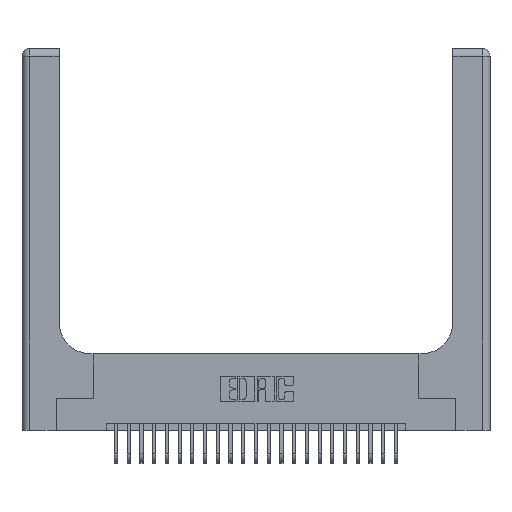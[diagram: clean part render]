
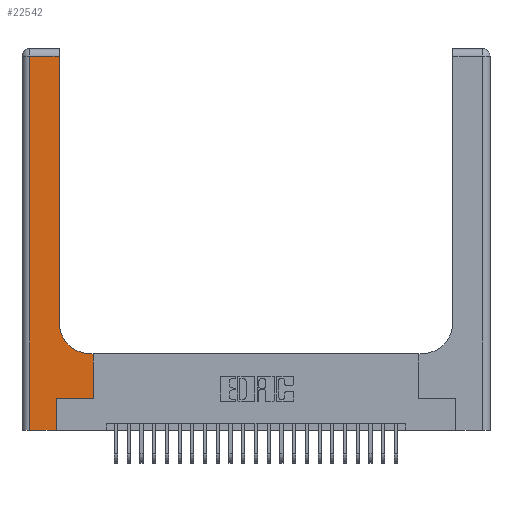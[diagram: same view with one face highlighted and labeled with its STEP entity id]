
A CAD part, top view. The second image highlights one B-rep face of the part: STEP entity #22542.
In plain terms, the highlighted planar face has unit normal (0, 0, 1).
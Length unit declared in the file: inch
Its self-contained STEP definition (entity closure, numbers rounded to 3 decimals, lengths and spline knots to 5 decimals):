
#578 = CARTESIAN_POINT ( 'NONE',  ( 0.2915, 3., 0.37 ) ) ;
#894 = CARTESIAN_POINT ( 'NONE',  ( 0.06, 0., 0.37 ) ) ;
#1270 = LINE ( 'NONE', #9552, #24621 ) ;
#1360 = VERTEX_POINT ( 'NONE', #11245 ) ;
#2136 = AXIS2_PLACEMENT_3D ( 'NONE', #14550, #2928, #16483 ) ;
#2551 = CARTESIAN_POINT ( 'NONE',  ( 0.5585, 0.6, 0.37 ) ) ;
#2597 = CARTESIAN_POINT ( 'NONE',  ( 0.2915, 0.6, 0.37 ) ) ;
#2928 = DIRECTION ( 'NONE',  ( 0., 0., -1. ) ) ;
#3600 = ORIENTED_EDGE ( 'NONE', *, *, #17276, .T. ) ;
#3623 = ORIENTED_EDGE ( 'NONE', *, *, #6206, .T. ) ;
#4839 = CARTESIAN_POINT ( 'NONE',  ( 0.269, 0.25, 0.37 ) ) ;
#5677 = CARTESIAN_POINT ( 'NONE',  ( 0.2915, 0.85, 0.37 ) ) ;
#5694 = DIRECTION ( 'NONE',  ( 1., 0., 0. ) ) ;
#5772 = EDGE_LOOP ( 'NONE', ( #7032, #15181, #12936, #11284, #8121, #16943, #3623, #3600, #11794 ) ) ;
#5927 = AXIS2_PLACEMENT_3D ( 'NONE', #22501, #10974, #24420 ) ;
#6032 = EDGE_CURVE ( 'NONE', #14086, #16810, #19579, .T. ) ;
#6108 = CIRCLE ( 'NONE', #5927, 0.25 ) ;
#6206 = EDGE_CURVE ( 'NONE', #20772, #7846, #21080, .T. ) ;
#6328 = LINE ( 'NONE', #6682, #21081 ) ;
#6501 = DIRECTION ( 'NONE',  ( 0., 1., 0. ) ) ;
#6682 = CARTESIAN_POINT ( 'NONE',  ( 0., 2.94, 0.37 ) ) ;
#7032 = ORIENTED_EDGE ( 'NONE', *, *, #6032, .T. ) ;
#7624 = CARTESIAN_POINT ( 'NONE',  ( 0.06, 2.94, 0.37 ) ) ;
#7846 = VERTEX_POINT ( 'NONE', #2551 ) ;
#8121 = ORIENTED_EDGE ( 'NONE', *, *, #21535, .T. ) ;
#8141 = VECTOR ( 'NONE', #14244, 39.37008 ) ;
#8176 = VERTEX_POINT ( 'NONE', #7624 ) ;
#8273 = CARTESIAN_POINT ( 'NONE',  ( 0.5585, 0.25, 0.37 ) ) ;
#9226 = CARTESIAN_POINT ( 'NONE',  ( 0.269, 0.25, 0.37 ) ) ;
#9552 = CARTESIAN_POINT ( 'NONE',  ( 0.06, 3., 0.37 ) ) ;
#9559 = VECTOR ( 'NONE', #14503, 39.37008 ) ;
#10638 = VECTOR ( 'NONE', #24788, 39.37008 ) ;
#10974 = DIRECTION ( 'NONE',  ( 0., 0., -1. ) ) ;
#11245 = CARTESIAN_POINT ( 'NONE',  ( 0.269, 0., 0.37 ) ) ;
#11254 = LINE ( 'NONE', #22874, #10638 ) ;
#11284 = ORIENTED_EDGE ( 'NONE', *, *, #15121, .T. ) ;
#11794 = ORIENTED_EDGE ( 'NONE', *, *, #15731, .T. ) ;
#12300 = VERTEX_POINT ( 'NONE', #9226 ) ;
#12328 = EDGE_CURVE ( 'NONE', #8176, #16740, #1270, .T. ) ;
#12769 = LINE ( 'NONE', #22939, #22420 ) ;
#12936 = ORIENTED_EDGE ( 'NONE', *, *, #12328, .T. ) ;
#13358 = VERTEX_POINT ( 'NONE', #14939 ) ;
#14086 = VERTEX_POINT ( 'NONE', #5677 ) ;
#14244 = DIRECTION ( 'NONE',  ( -1., 0., 0. ) ) ;
#14503 = DIRECTION ( 'NONE',  ( 1., 0., 0. ) ) ;
#14550 = CARTESIAN_POINT ( 'NONE',  ( 0., 3., 0.37 ) ) ;
#14642 = DIRECTION ( 'NONE',  ( 0., 1., 0. ) ) ;
#14939 = CARTESIAN_POINT ( 'NONE',  ( 0.5415, 0.6, 0.37 ) ) ;
#15121 = EDGE_CURVE ( 'NONE', #16740, #1360, #12769, .T. ) ;
#15181 = ORIENTED_EDGE ( 'NONE', *, *, #17351, .T. ) ;
#15340 = VECTOR ( 'NONE', #14642, 39.37008 ) ;
#15731 = EDGE_CURVE ( 'NONE', #13358, #14086, #6108, .T. ) ;
#15873 = LINE ( 'NONE', #4839, #9559 ) ;
#16345 = DIRECTION ( 'NONE',  ( -1., 0., 0. ) ) ;
#16483 = DIRECTION ( 'NONE',  ( -1., 0., 0. ) ) ;
#16569 = CARTESIAN_POINT ( 'NONE',  ( 0.5585, 0.25, 0.37 ) ) ;
#16740 = VERTEX_POINT ( 'NONE', #894 ) ;
#16810 = VERTEX_POINT ( 'NONE', #20490 ) ;
#16943 = ORIENTED_EDGE ( 'NONE', *, *, #23669, .T. ) ;
#17276 = EDGE_CURVE ( 'NONE', #7846, #13358, #22309, .T. ) ;
#17351 = EDGE_CURVE ( 'NONE', #16810, #8176, #6328, .T. ) ;
#19141 = DIRECTION ( 'NONE',  ( 0., -1., 0. ) ) ;
#19579 = LINE ( 'NONE', #578, #24092 ) ;
#20292 = PLANE ( 'NONE',  #2136 ) ;
#20490 = CARTESIAN_POINT ( 'NONE',  ( 0.2915, 2.94, 0.37 ) ) ;
#20772 = VERTEX_POINT ( 'NONE', #8273 ) ;
#21080 = LINE ( 'NONE', #16569, #15340 ) ;
#21081 = VECTOR ( 'NONE', #16345, 39.37008 ) ;
#21535 = EDGE_CURVE ( 'NONE', #1360, #12300, #11254, .T. ) ;
#22309 = LINE ( 'NONE', #2597, #8141 ) ;
#22420 = VECTOR ( 'NONE', #5694, 39.37008 ) ;
#22501 = CARTESIAN_POINT ( 'NONE',  ( 0.5415, 0.85, 0.37 ) ) ;
#22542 = ADVANCED_FACE ( 'NONE', ( #24468 ), #20292, .F. ) ;
#22874 = CARTESIAN_POINT ( 'NONE',  ( 0.269, 0., 0.37 ) ) ;
#22939 = CARTESIAN_POINT ( 'NONE',  ( 0., 0., 0.37 ) ) ;
#23669 = EDGE_CURVE ( 'NONE', #12300, #20772, #15873, .T. ) ;
#24092 = VECTOR ( 'NONE', #6501, 39.37008 ) ;
#24420 = DIRECTION ( 'NONE',  ( 1., 0., 0. ) ) ;
#24468 = FACE_OUTER_BOUND ( 'NONE', #5772, .T. ) ;
#24621 = VECTOR ( 'NONE', #19141, 39.37008 ) ;
#24788 = DIRECTION ( 'NONE',  ( 0., 1., 0. ) ) ;
